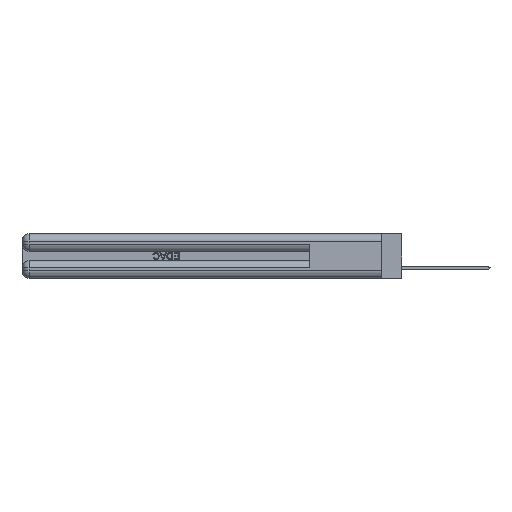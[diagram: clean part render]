
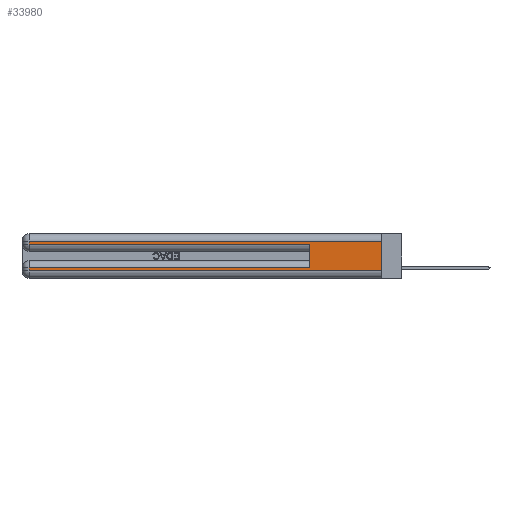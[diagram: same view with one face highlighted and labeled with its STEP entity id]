
A CAD part, left-side view. The second image highlights one B-rep face of the part: STEP entity #33980.
In plain terms, the highlighted planar face has unit normal (-1, 0, 0).
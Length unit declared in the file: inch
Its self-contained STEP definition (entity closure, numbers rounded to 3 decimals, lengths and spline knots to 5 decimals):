
#307 = VERTEX_POINT ( 'NONE', #32454 ) ;
#962 = FACE_OUTER_BOUND ( 'NONE', #11769, .T. ) ;
#2682 = VERTEX_POINT ( 'NONE', #39024 ) ;
#3925 = LINE ( 'NONE', #12183, #16116 ) ;
#4415 = LINE ( 'NONE', #34188, #40469 ) ;
#4676 = VECTOR ( 'NONE', #42176, 39.37008 ) ;
#5300 = ORIENTED_EDGE ( 'NONE', *, *, #13806, .T. ) ;
#8136 = EDGE_CURVE ( 'NONE', #15628, #19037, #39466, .T. ) ;
#9317 = CARTESIAN_POINT ( 'NONE',  ( 0., 0., 0.06 ) ) ;
#10730 = LINE ( 'NONE', #43501, #41255 ) ;
#11418 = ORIENTED_EDGE ( 'NONE', *, *, #24336, .T. ) ;
#11707 = CARTESIAN_POINT ( 'NONE',  ( 0., 0., 0.37 ) ) ;
#11769 = EDGE_LOOP ( 'NONE', ( #34558, #26669, #15905, #5300, #20694, #38724, #11418, #42365 ) ) ;
#11942 = LINE ( 'NONE', #12516, #21956 ) ;
#12003 = CARTESIAN_POINT ( 'NONE',  ( 0., 2.94, 0.285 ) ) ;
#12015 = DIRECTION ( 'NONE',  ( 0., 1., 0. ) ) ;
#12183 = CARTESIAN_POINT ( 'NONE',  ( 0., 0., 0.085 ) ) ;
#12516 = CARTESIAN_POINT ( 'NONE',  ( 0., 2.94, 0.37 ) ) ;
#12902 = DIRECTION ( 'NONE',  ( 0., -1., 0. ) ) ;
#13806 = EDGE_CURVE ( 'NONE', #36427, #2682, #41038, .T. ) ;
#15478 = CARTESIAN_POINT ( 'NONE',  ( 0., 2.94, 0.085 ) ) ;
#15628 = VERTEX_POINT ( 'NONE', #17849 ) ;
#15896 = EDGE_CURVE ( 'NONE', #15628, #22443, #37470, .T. ) ;
#15905 = ORIENTED_EDGE ( 'NONE', *, *, #38705, .T. ) ;
#16116 = VECTOR ( 'NONE', #12015, 39.37008 ) ;
#17849 = CARTESIAN_POINT ( 'NONE',  ( 0., 0., 0.31 ) ) ;
#18565 = LINE ( 'NONE', #19112, #41997 ) ;
#19037 = VERTEX_POINT ( 'NONE', #9317 ) ;
#19112 = CARTESIAN_POINT ( 'NONE',  ( 0., 0.6, 0.145 ) ) ;
#19857 = DIRECTION ( 'NONE',  ( 0., 0., -1. ) ) ;
#20694 = ORIENTED_EDGE ( 'NONE', *, *, #25919, .F. ) ;
#21956 = VECTOR ( 'NONE', #40913, 39.37008 ) ;
#22186 = DIRECTION ( 'NONE',  ( 0., 0., -1. ) ) ;
#22443 = VERTEX_POINT ( 'NONE', #25470 ) ;
#24336 = EDGE_CURVE ( 'NONE', #37434, #307, #10730, .T. ) ;
#25470 = CARTESIAN_POINT ( 'NONE',  ( 0., 2.94, 0.31 ) ) ;
#25919 = EDGE_CURVE ( 'NONE', #41851, #2682, #18565, .T. ) ;
#26669 = ORIENTED_EDGE ( 'NONE', *, *, #15896, .T. ) ;
#29283 = EDGE_CURVE ( 'NONE', #41851, #37434, #3925, .T. ) ;
#29965 = EDGE_CURVE ( 'NONE', #307, #19037, #4415, .T. ) ;
#32454 = CARTESIAN_POINT ( 'NONE',  ( 0., 2.94, 0.06 ) ) ;
#33861 = VECTOR ( 'NONE', #41269, 39.37008 ) ;
#33980 = ADVANCED_FACE ( 'NONE', ( #962 ), #39584, .F. ) ;
#34188 = CARTESIAN_POINT ( 'NONE',  ( 0., 0., 0.06 ) ) ;
#34558 = ORIENTED_EDGE ( 'NONE', *, *, #8136, .F. ) ;
#36427 = VERTEX_POINT ( 'NONE', #12003 ) ;
#36643 = CARTESIAN_POINT ( 'NONE',  ( 0., 0., 0.37 ) ) ;
#37078 = CARTESIAN_POINT ( 'NONE',  ( 0., 0.6, 0.085 ) ) ;
#37264 = VECTOR ( 'NONE', #43369, 39.37008 ) ;
#37382 = CARTESIAN_POINT ( 'NONE',  ( 0., 0., 0.285 ) ) ;
#37434 = VERTEX_POINT ( 'NONE', #15478 ) ;
#37470 = LINE ( 'NONE', #37481, #4676 ) ;
#37481 = CARTESIAN_POINT ( 'NONE',  ( 0., 0., 0.31 ) ) ;
#38705 = EDGE_CURVE ( 'NONE', #22443, #36427, #11942, .T. ) ;
#38724 = ORIENTED_EDGE ( 'NONE', *, *, #29283, .T. ) ;
#39024 = CARTESIAN_POINT ( 'NONE',  ( 0., 0.6, 0.285 ) ) ;
#39466 = LINE ( 'NONE', #11707, #37264 ) ;
#39584 = PLANE ( 'NONE',  #44126 ) ;
#40469 = VECTOR ( 'NONE', #12902, 39.37008 ) ;
#40913 = DIRECTION ( 'NONE',  ( 0., 0., -1. ) ) ;
#41038 = LINE ( 'NONE', #37382, #33861 ) ;
#41255 = VECTOR ( 'NONE', #19857, 39.37008 ) ;
#41269 = DIRECTION ( 'NONE',  ( 0., -1., 0. ) ) ;
#41851 = VERTEX_POINT ( 'NONE', #37078 ) ;
#41997 = VECTOR ( 'NONE', #43805, 39.37008 ) ;
#42176 = DIRECTION ( 'NONE',  ( 0., 1., 0. ) ) ;
#42365 = ORIENTED_EDGE ( 'NONE', *, *, #29965, .T. ) ;
#43028 = DIRECTION ( 'NONE',  ( 1., 0., 0. ) ) ;
#43369 = DIRECTION ( 'NONE',  ( 0., 0., -1. ) ) ;
#43501 = CARTESIAN_POINT ( 'NONE',  ( 0., 2.94, 0.37 ) ) ;
#43805 = DIRECTION ( 'NONE',  ( 0., 0., 1. ) ) ;
#44126 = AXIS2_PLACEMENT_3D ( 'NONE', #36643, #43028, #22186 ) ;
